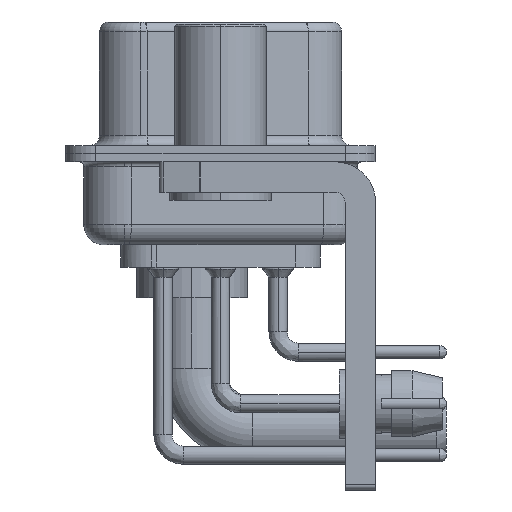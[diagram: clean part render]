
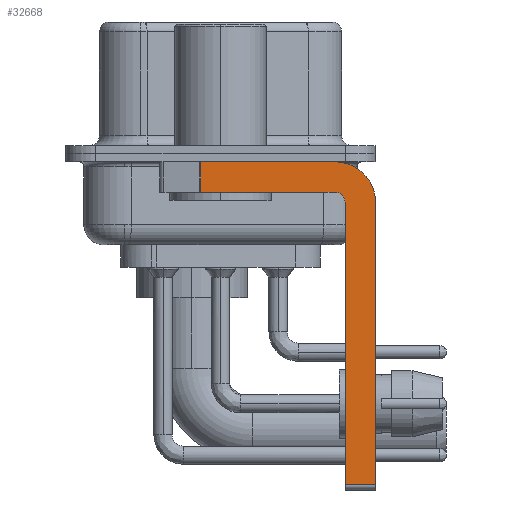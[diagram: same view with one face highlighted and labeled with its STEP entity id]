
A CAD part, left-side view. The second image highlights one B-rep face of the part: STEP entity #32668.
In plain terms, the highlighted planar face has unit normal (-1, 0, 0).
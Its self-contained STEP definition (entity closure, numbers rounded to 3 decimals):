
#284 = CARTESIAN_POINT ( 'NONE',  ( -2.9, -5.65, -0.4 ) ) ;
#1784 = DIRECTION ( 'NONE',  ( 0., 0., -1. ) ) ;
#1972 = VERTEX_POINT ( 'NONE', #25080 ) ;
#2684 = ORIENTED_EDGE ( 'NONE', *, *, #9161, .F. ) ;
#3693 = EDGE_CURVE ( 'NONE', #17657, #7401, #19014, .T. ) ;
#3783 = DIRECTION ( 'NONE',  ( 0., 0., 1. ) ) ;
#3803 = ORIENTED_EDGE ( 'NONE', *, *, #40307, .F. ) ;
#4640 = CARTESIAN_POINT ( 'NONE',  ( -2.9, 0.978, -1.9 ) ) ;
#4936 = ORIENTED_EDGE ( 'NONE', *, *, #5435, .F. ) ;
#5075 = CARTESIAN_POINT ( 'NONE',  ( -2.9, -7.65, -2.4 ) ) ;
#5435 = EDGE_CURVE ( 'NONE', #1972, #31018, #33461, .T. ) ;
#6325 = CARTESIAN_POINT ( 'NONE',  ( -2.9, -5.65, -2.4 ) ) ;
#7401 = VERTEX_POINT ( 'NONE', #284 ) ;
#7448 = LINE ( 'NONE', #13072, #30991 ) ;
#9077 = DIRECTION ( 'NONE',  ( 0., -1., 0. ) ) ;
#9161 = EDGE_CURVE ( 'NONE', #17830, #24022, #18629, .T. ) ;
#10110 = DIRECTION ( 'NONE',  ( 0., -1., 0. ) ) ;
#10928 = DIRECTION ( 'NONE',  ( 1., 0., 0. ) ) ;
#12024 = LINE ( 'NONE', #4640, #19509 ) ;
#12297 = ORIENTED_EDGE ( 'NONE', *, *, #3693, .F. ) ;
#13072 = CARTESIAN_POINT ( 'NONE',  ( -2.9, -5.65, -1.9 ) ) ;
#13148 = EDGE_CURVE ( 'NONE', #17657, #15151, #12024, .T. ) ;
#15147 = CARTESIAN_POINT ( 'NONE',  ( -2.9, -6.15, -2.4 ) ) ;
#15151 = VERTEX_POINT ( 'NONE', #20641 ) ;
#15985 = DIRECTION ( 'NONE',  ( 0., 0., 1. ) ) ;
#16153 = ORIENTED_EDGE ( 'NONE', *, *, #37268, .T. ) ;
#16253 = DIRECTION ( 'NONE',  ( 1., 0., 0. ) ) ;
#16380 = DIRECTION ( 'NONE',  ( 0., 1., 0. ) ) ;
#16405 = EDGE_CURVE ( 'NONE', #24022, #15151, #7448, .T. ) ;
#16594 = DIRECTION ( 'NONE',  ( -1., 0., 0. ) ) ;
#16625 = AXIS2_PLACEMENT_3D ( 'NONE', #22626, #16594, #3783 ) ;
#17657 = VERTEX_POINT ( 'NONE', #35289 ) ;
#17830 = VERTEX_POINT ( 'NONE', #15147 ) ;
#18356 = ORIENTED_EDGE ( 'NONE', *, *, #13148, .T. ) ;
#18629 = CIRCLE ( 'NONE', #16625, 0.5 ) ;
#19014 = LINE ( 'NONE', #35176, #30599 ) ;
#19509 = VECTOR ( 'NONE', #31106, 1000. ) ;
#20641 = CARTESIAN_POINT ( 'NONE',  ( -2.9, 0.978, -1.9 ) ) ;
#20838 = EDGE_CURVE ( 'NONE', #31776, #17830, #25321, .T. ) ;
#21799 = AXIS2_PLACEMENT_3D ( 'NONE', #6325, #16253, #32229 ) ;
#22626 = CARTESIAN_POINT ( 'NONE',  ( -2.9, -5.65, -2.4 ) ) ;
#22757 = CARTESIAN_POINT ( 'NONE',  ( -2.9, -5.65, -16.35 ) ) ;
#24022 = VERTEX_POINT ( 'NONE', #34032 ) ;
#24195 = CARTESIAN_POINT ( 'NONE',  ( -2.9, -7.65, -16.35 ) ) ;
#24451 = LINE ( 'NONE', #22757, #39728 ) ;
#24966 = VECTOR ( 'NONE', #1784, 1000. ) ;
#25080 = CARTESIAN_POINT ( 'NONE',  ( -2.9, -7.65, -2.4 ) ) ;
#25321 = LINE ( 'NONE', #29049, #31474 ) ;
#25359 = ORIENTED_EDGE ( 'NONE', *, *, #16405, .F. ) ;
#26023 = CIRCLE ( 'NONE', #31330, 2. ) ;
#29049 = CARTESIAN_POINT ( 'NONE',  ( -2.9, -6.15, -16.6 ) ) ;
#29804 = CARTESIAN_POINT ( 'NONE',  ( -2.9, -5.65, -2.4 ) ) ;
#29935 = EDGE_LOOP ( 'NONE', ( #12297, #18356, #25359, #2684, #36336, #16153, #4936, #3803 ) ) ;
#30599 = VECTOR ( 'NONE', #9077, 1000. ) ;
#30991 = VECTOR ( 'NONE', #16380, 1000. ) ;
#31018 = VERTEX_POINT ( 'NONE', #24195 ) ;
#31106 = DIRECTION ( 'NONE',  ( 0., 0., -1. ) ) ;
#31330 = AXIS2_PLACEMENT_3D ( 'NONE', #29804, #10928, #33127 ) ;
#31474 = VECTOR ( 'NONE', #15985, 1000. ) ;
#31776 = VERTEX_POINT ( 'NONE', #38194 ) ;
#32229 = DIRECTION ( 'NONE',  ( 0., 0., -1. ) ) ;
#32668 = ADVANCED_FACE ( 'NONE', ( #35138 ), #35543, .F. ) ;
#33127 = DIRECTION ( 'NONE',  ( 0., 0., -1. ) ) ;
#33461 = LINE ( 'NONE', #5075, #24966 ) ;
#34032 = CARTESIAN_POINT ( 'NONE',  ( -2.9, -5.65, -1.9 ) ) ;
#35138 = FACE_OUTER_BOUND ( 'NONE', #29935, .T. ) ;
#35176 = CARTESIAN_POINT ( 'NONE',  ( -2.9, 3., -0.4 ) ) ;
#35289 = CARTESIAN_POINT ( 'NONE',  ( -2.9, 0.978, -0.4 ) ) ;
#35543 = PLANE ( 'NONE',  #21799 ) ;
#36336 = ORIENTED_EDGE ( 'NONE', *, *, #20838, .F. ) ;
#37268 = EDGE_CURVE ( 'NONE', #31776, #31018, #24451, .T. ) ;
#38194 = CARTESIAN_POINT ( 'NONE',  ( -2.9, -6.15, -16.35 ) ) ;
#39728 = VECTOR ( 'NONE', #10110, 1000. ) ;
#40307 = EDGE_CURVE ( 'NONE', #7401, #1972, #26023, .T. ) ;
